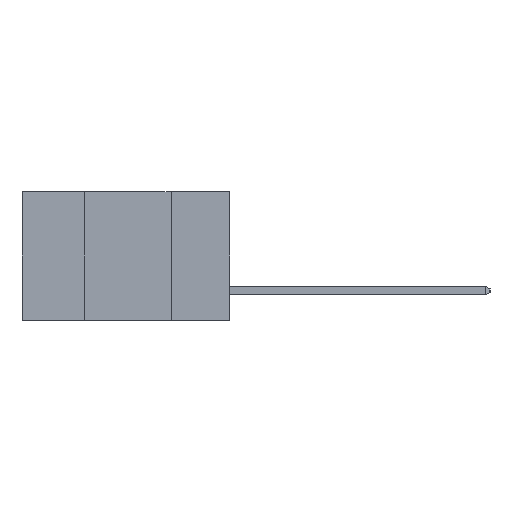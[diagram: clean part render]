
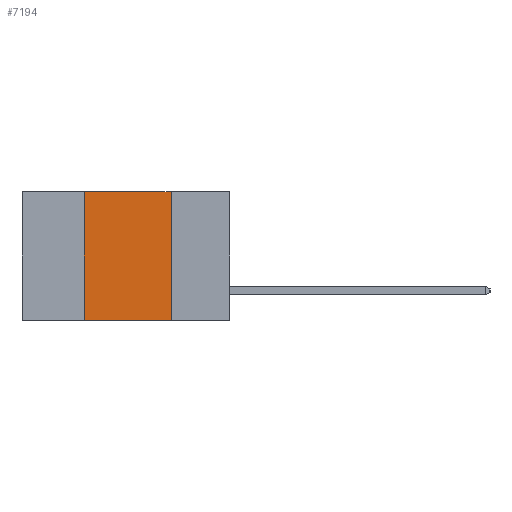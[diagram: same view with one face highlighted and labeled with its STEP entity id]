
A CAD part, left-side view. The second image highlights one B-rep face of the part: STEP entity #7194.
In plain terms, the highlighted planar face has unit normal (-1, 0, 0).
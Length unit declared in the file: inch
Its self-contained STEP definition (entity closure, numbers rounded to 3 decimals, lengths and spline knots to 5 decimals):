
#404 = CARTESIAN_POINT ( 'NONE',  ( 0., 0.42, -0.37 ) ) ;
#584 = VERTEX_POINT ( 'NONE', #7030 ) ;
#1064 = EDGE_CURVE ( 'NONE', #1152, #584, #2387, .T. ) ;
#1152 = VERTEX_POINT ( 'NONE', #8434 ) ;
#1562 = VECTOR ( 'NONE', #1725, 39.37008 ) ;
#1578 = VERTEX_POINT ( 'NONE', #1935 ) ;
#1725 = DIRECTION ( 'NONE',  ( 0., 0., -1. ) ) ;
#1799 = VECTOR ( 'NONE', #6613, 39.37008 ) ;
#1834 = DIRECTION ( 'NONE',  ( 0., -1., 0. ) ) ;
#1907 = CARTESIAN_POINT ( 'NONE',  ( 0., 0.6, -0.37 ) ) ;
#1935 = CARTESIAN_POINT ( 'NONE',  ( 0., 0.42, -0.37 ) ) ;
#2387 = LINE ( 'NONE', #7339, #6205 ) ;
#2933 = EDGE_CURVE ( 'NONE', #1578, #6536, #9394, .T. ) ;
#2976 = FACE_OUTER_BOUND ( 'NONE', #4598, .T. ) ;
#3024 = CARTESIAN_POINT ( 'NONE',  ( 0., 0.6, 0. ) ) ;
#3664 = VECTOR ( 'NONE', #1834, 39.37008 ) ;
#3788 = DIRECTION ( 'NONE',  ( 0., 0., -1. ) ) ;
#4065 = CARTESIAN_POINT ( 'NONE',  ( 0., 0.17, -0.37 ) ) ;
#4598 = EDGE_LOOP ( 'NONE', ( #9118, #4657, #8393, #5024 ) ) ;
#4657 = ORIENTED_EDGE ( 'NONE', *, *, #1064, .F. ) ;
#5024 = ORIENTED_EDGE ( 'NONE', *, *, #2933, .T. ) ;
#6119 = DIRECTION ( 'NONE',  ( 0., -1., 0. ) ) ;
#6160 = LINE ( 'NONE', #404, #1799 ) ;
#6205 = VECTOR ( 'NONE', #6119, 39.37008 ) ;
#6444 = AXIS2_PLACEMENT_3D ( 'NONE', #3024, #8174, #3788 ) ;
#6536 = VERTEX_POINT ( 'NONE', #8998 ) ;
#6613 = DIRECTION ( 'NONE',  ( 0., 0., 1. ) ) ;
#7030 = CARTESIAN_POINT ( 'NONE',  ( 0., 0.17, 0. ) ) ;
#7194 = ADVANCED_FACE ( 'NONE', ( #2976 ), #7458, .F. ) ;
#7339 = CARTESIAN_POINT ( 'NONE',  ( 0., 0.6, 0. ) ) ;
#7458 = PLANE ( 'NONE',  #6444 ) ;
#7958 = EDGE_CURVE ( 'NONE', #584, #6536, #9424, .T. ) ;
#8174 = DIRECTION ( 'NONE',  ( 1., 0., 0. ) ) ;
#8393 = ORIENTED_EDGE ( 'NONE', *, *, #8816, .F. ) ;
#8434 = CARTESIAN_POINT ( 'NONE',  ( 0., 0.42, 0. ) ) ;
#8816 = EDGE_CURVE ( 'NONE', #1578, #1152, #6160, .T. ) ;
#8998 = CARTESIAN_POINT ( 'NONE',  ( 0., 0.17, -0.37 ) ) ;
#9118 = ORIENTED_EDGE ( 'NONE', *, *, #7958, .F. ) ;
#9394 = LINE ( 'NONE', #1907, #3664 ) ;
#9424 = LINE ( 'NONE', #4065, #1562 ) ;
